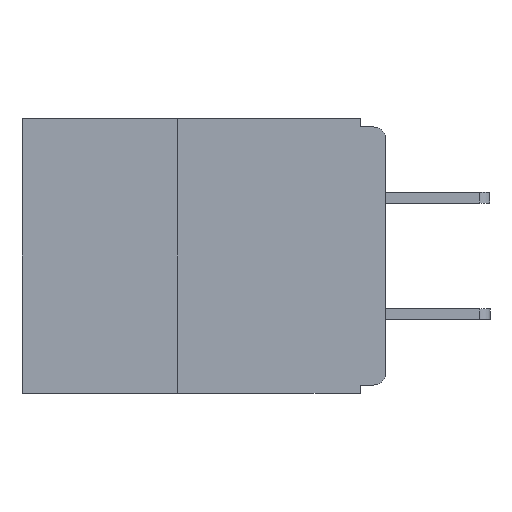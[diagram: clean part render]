
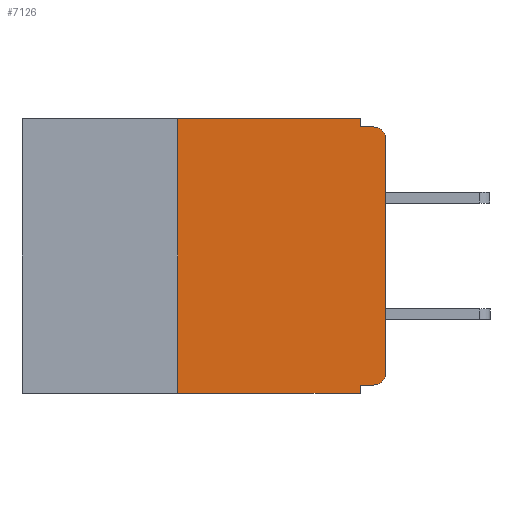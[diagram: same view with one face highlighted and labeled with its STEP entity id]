
A CAD part, left-side view. The second image highlights one B-rep face of the part: STEP entity #7126.
In plain terms, the highlighted planar face has unit normal (-1, 0, 0).
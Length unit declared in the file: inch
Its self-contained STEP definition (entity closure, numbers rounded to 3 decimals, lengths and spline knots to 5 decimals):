
#311 = DIRECTION ( 'NONE',  ( -1., 0., 0. ) ) ;
#354 = CARTESIAN_POINT ( 'NONE',  ( 0., 0.015, -0.32 ) ) ;
#389 = LINE ( 'NONE', #5583, #11896 ) ;
#395 = VERTEX_POINT ( 'NONE', #2533 ) ;
#478 = VERTEX_POINT ( 'NONE', #6172 ) ;
#486 = VERTEX_POINT ( 'NONE', #6622 ) ;
#667 = DIRECTION ( 'NONE',  ( 0., -1., 0. ) ) ;
#1149 = LINE ( 'NONE', #12366, #9783 ) ;
#1177 = ORIENTED_EDGE ( 'NONE', *, *, #11263, .T. ) ;
#1253 = VERTEX_POINT ( 'NONE', #12843 ) ;
#1306 = VECTOR ( 'NONE', #9212, 39.37008 ) ;
#1368 = EDGE_CURVE ( 'NONE', #7720, #486, #11189, .T. ) ;
#1531 = EDGE_LOOP ( 'NONE', ( #2830, #11604, #3149, #6180, #11929, #3526, #12265, #3916, #6899, #1177 ) ) ;
#1815 = EDGE_CURVE ( 'NONE', #486, #1253, #12953, .T. ) ;
#2533 = CARTESIAN_POINT ( 'NONE',  ( 0., 0.25, -0.33 ) ) ;
#2830 = ORIENTED_EDGE ( 'NONE', *, *, #11181, .T. ) ;
#3107 = AXIS2_PLACEMENT_3D ( 'NONE', #4755, #4659, #4652 ) ;
#3149 = ORIENTED_EDGE ( 'NONE', *, *, #8584, .F. ) ;
#3440 = AXIS2_PLACEMENT_3D ( 'NONE', #7187, #311, #8269 ) ;
#3526 = ORIENTED_EDGE ( 'NONE', *, *, #12439, .F. ) ;
#3620 = DIRECTION ( 'NONE',  ( 0., 0., 1. ) ) ;
#3699 = VECTOR ( 'NONE', #8858, 39.37008 ) ;
#3916 = ORIENTED_EDGE ( 'NONE', *, *, #13803, .F. ) ;
#4432 = CARTESIAN_POINT ( 'NONE',  ( 0., 0., -0.01 ) ) ;
#4652 = DIRECTION ( 'NONE',  ( 0., 0., -1. ) ) ;
#4659 = DIRECTION ( 'NONE',  ( 1., 0., 0. ) ) ;
#4694 = PLANE ( 'NONE',  #3107 ) ;
#4755 = CARTESIAN_POINT ( 'NONE',  ( 0., 0.437, 0. ) ) ;
#4879 = CARTESIAN_POINT ( 'NONE',  ( 0., 0.015, -0.01 ) ) ;
#5114 = AXIS2_PLACEMENT_3D ( 'NONE', #8672, #8670, #8795 ) ;
#5137 = EDGE_CURVE ( 'NONE', #6938, #7104, #13709, .T. ) ;
#5583 = CARTESIAN_POINT ( 'NONE',  ( 0., 0.437, -0.33 ) ) ;
#5854 = CARTESIAN_POINT ( 'NONE',  ( 0., 0.25, -0.33 ) ) ;
#6104 = CARTESIAN_POINT ( 'NONE',  ( 0., 0., -0.025 ) ) ;
#6150 = CIRCLE ( 'NONE', #3440, 0.015 ) ;
#6172 = CARTESIAN_POINT ( 'NONE',  ( 0., 0.031, -0.33 ) ) ;
#6180 = ORIENTED_EDGE ( 'NONE', *, *, #1815, .F. ) ;
#6342 = CARTESIAN_POINT ( 'NONE',  ( 0., 0.437, 0. ) ) ;
#6384 = VERTEX_POINT ( 'NONE', #10388 ) ;
#6622 = CARTESIAN_POINT ( 'NONE',  ( 0., 0.031, 0. ) ) ;
#6846 = CARTESIAN_POINT ( 'NONE',  ( 0., 0.031, -0.33 ) ) ;
#6899 = ORIENTED_EDGE ( 'NONE', *, *, #11000, .F. ) ;
#6938 = VERTEX_POINT ( 'NONE', #6104 ) ;
#7104 = VERTEX_POINT ( 'NONE', #4879 ) ;
#7106 = CARTESIAN_POINT ( 'NONE',  ( 0., 0., -0.305 ) ) ;
#7126 = ADVANCED_FACE ( 'NONE', ( #8232 ), #4694, .F. ) ;
#7187 = CARTESIAN_POINT ( 'NONE',  ( 0., 0.015, -0.305 ) ) ;
#7720 = VERTEX_POINT ( 'NONE', #13699 ) ;
#7842 = LINE ( 'NONE', #6846, #13143 ) ;
#8232 = FACE_OUTER_BOUND ( 'NONE', #1531, .T. ) ;
#8269 = DIRECTION ( 'NONE',  ( 0., 0., -1. ) ) ;
#8584 = EDGE_CURVE ( 'NONE', #1253, #7104, #11527, .T. ) ;
#8670 = DIRECTION ( 'NONE',  ( -1., 0., 0. ) ) ;
#8672 = CARTESIAN_POINT ( 'NONE',  ( 0., 0.015, -0.025 ) ) ;
#8691 = VECTOR ( 'NONE', #667, 39.37008 ) ;
#8705 = VECTOR ( 'NONE', #8840, 39.37008 ) ;
#8795 = DIRECTION ( 'NONE',  ( 0., 0., -1. ) ) ;
#8840 = DIRECTION ( 'NONE',  ( 0., -1., 0. ) ) ;
#8858 = DIRECTION ( 'NONE',  ( 0., 1., 0. ) ) ;
#8879 = DIRECTION ( 'NONE',  ( 0., 0., -1. ) ) ;
#8934 = DIRECTION ( 'NONE',  ( 0., -1., 0. ) ) ;
#9212 = DIRECTION ( 'NONE',  ( 0., 0., 1. ) ) ;
#9783 = VECTOR ( 'NONE', #3620, 39.37008 ) ;
#10143 = DIRECTION ( 'NONE',  ( 0., 0., -1. ) ) ;
#10200 = VECTOR ( 'NONE', #8879, 39.37008 ) ;
#10388 = CARTESIAN_POINT ( 'NONE',  ( 0., 0.031, -0.32 ) ) ;
#10678 = CARTESIAN_POINT ( 'NONE',  ( 0., 0.031, 0. ) ) ;
#10725 = VERTEX_POINT ( 'NONE', #7106 ) ;
#10999 = CARTESIAN_POINT ( 'NONE',  ( 0., 0., -0.32 ) ) ;
#11000 = EDGE_CURVE ( 'NONE', #11287, #6384, #12408, .T. ) ;
#11181 = EDGE_CURVE ( 'NONE', #10725, #6938, #1149, .T. ) ;
#11189 = LINE ( 'NONE', #6342, #8691 ) ;
#11263 = EDGE_CURVE ( 'NONE', #11287, #10725, #6150, .T. ) ;
#11287 = VERTEX_POINT ( 'NONE', #354 ) ;
#11527 = LINE ( 'NONE', #4432, #8705 ) ;
#11604 = ORIENTED_EDGE ( 'NONE', *, *, #5137, .T. ) ;
#11649 = EDGE_CURVE ( 'NONE', #395, #478, #389, .T. ) ;
#11896 = VECTOR ( 'NONE', #8934, 39.37008 ) ;
#11929 = ORIENTED_EDGE ( 'NONE', *, *, #1368, .F. ) ;
#12265 = ORIENTED_EDGE ( 'NONE', *, *, #11649, .T. ) ;
#12366 = CARTESIAN_POINT ( 'NONE',  ( 0., 0., 0. ) ) ;
#12408 = LINE ( 'NONE', #10999, #3699 ) ;
#12439 = EDGE_CURVE ( 'NONE', #395, #7720, #13021, .T. ) ;
#12843 = CARTESIAN_POINT ( 'NONE',  ( 0., 0.031, -0.01 ) ) ;
#12953 = LINE ( 'NONE', #10678, #10200 ) ;
#13021 = LINE ( 'NONE', #5854, #1306 ) ;
#13143 = VECTOR ( 'NONE', #10143, 39.37008 ) ;
#13699 = CARTESIAN_POINT ( 'NONE',  ( 0., 0.25, 0. ) ) ;
#13709 = CIRCLE ( 'NONE', #5114, 0.015 ) ;
#13803 = EDGE_CURVE ( 'NONE', #6384, #478, #7842, .T. ) ;
